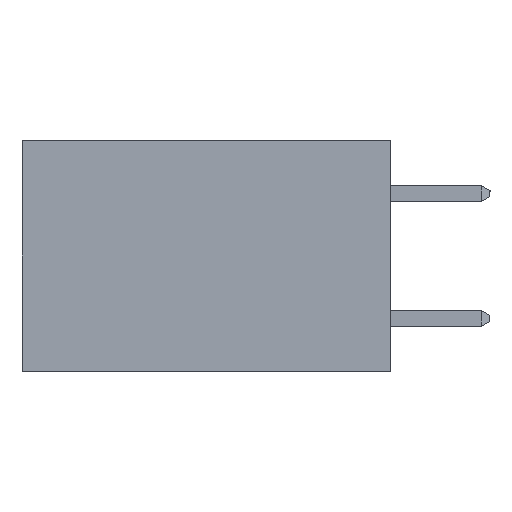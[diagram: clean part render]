
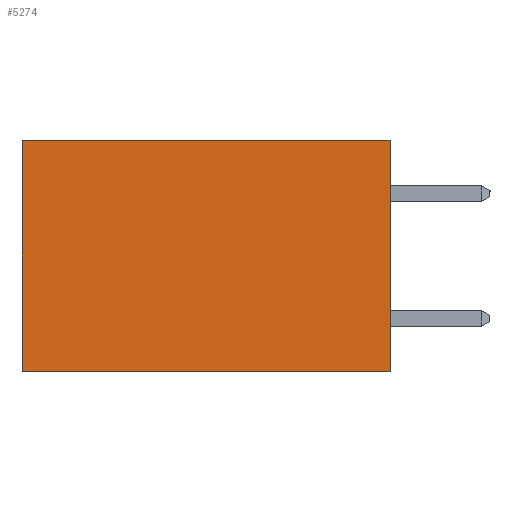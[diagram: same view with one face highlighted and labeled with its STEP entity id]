
A CAD part, left-side view. The second image highlights one B-rep face of the part: STEP entity #5274.
In plain terms, the highlighted planar face has unit normal (-1, 0, 0).
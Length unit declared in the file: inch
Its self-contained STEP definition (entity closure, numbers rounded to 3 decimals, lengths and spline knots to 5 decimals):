
#259 = AXIS2_PLACEMENT_3D ( 'NONE', #12889, #12872, #12855 ) ;
#448 = CARTESIAN_POINT ( 'NONE',  ( 0.277, 0., 0. ) ) ;
#1211 = CARTESIAN_POINT ( 'NONE',  ( 0.277, 0.59, -0.37 ) ) ;
#1327 = EDGE_CURVE ( 'NONE', #5012, #11931, #10814, .T. ) ;
#2160 = EDGE_CURVE ( 'NONE', #11732, #11931, #6467, .T. ) ;
#2224 = ORIENTED_EDGE ( 'NONE', *, *, #1327, .F. ) ;
#2859 = DIRECTION ( 'NONE',  ( 0., 0., -1. ) ) ;
#3295 = EDGE_CURVE ( 'NONE', #13383, #5012, #11925, .T. ) ;
#3427 = CARTESIAN_POINT ( 'NONE',  ( 0.277, 0., -0.37 ) ) ;
#3452 = VECTOR ( 'NONE', #5341, 39.37008 ) ;
#3550 = FACE_OUTER_BOUND ( 'NONE', #4337, .T. ) ;
#4129 = CARTESIAN_POINT ( 'NONE',  ( 0.277, 0.59, 0. ) ) ;
#4337 = EDGE_LOOP ( 'NONE', ( #13172, #2224, #5355, #5174 ) ) ;
#4880 = EDGE_CURVE ( 'NONE', #13383, #11732, #12362, .T. ) ;
#5012 = VERTEX_POINT ( 'NONE', #10967 ) ;
#5174 = ORIENTED_EDGE ( 'NONE', *, *, #4880, .T. ) ;
#5274 = ADVANCED_FACE ( 'NONE', ( #3550 ), #13047, .F. ) ;
#5341 = DIRECTION ( 'NONE',  ( 0., 0., -1. ) ) ;
#5355 = ORIENTED_EDGE ( 'NONE', *, *, #3295, .F. ) ;
#5693 = CARTESIAN_POINT ( 'NONE',  ( 0.277, 0.59, -0.37 ) ) ;
#5754 = VECTOR ( 'NONE', #2859, 39.37008 ) ;
#6467 = LINE ( 'NONE', #5693, #5754 ) ;
#8278 = DIRECTION ( 'NONE',  ( 0., 1., 0. ) ) ;
#8543 = VECTOR ( 'NONE', #8278, 39.37008 ) ;
#10172 = CARTESIAN_POINT ( 'NONE',  ( 0.277, 0., -0.37 ) ) ;
#10472 = VECTOR ( 'NONE', #10936, 39.37008 ) ;
#10814 = LINE ( 'NONE', #10172, #10472 ) ;
#10936 = DIRECTION ( 'NONE',  ( 0., 1., 0. ) ) ;
#10967 = CARTESIAN_POINT ( 'NONE',  ( 0.277, 0., -0.37 ) ) ;
#11732 = VERTEX_POINT ( 'NONE', #4129 ) ;
#11925 = LINE ( 'NONE', #3427, #3452 ) ;
#11931 = VERTEX_POINT ( 'NONE', #1211 ) ;
#12362 = LINE ( 'NONE', #448, #8543 ) ;
#12855 = DIRECTION ( 'NONE',  ( 0., 0., -1. ) ) ;
#12872 = DIRECTION ( 'NONE',  ( 1., 0., 0. ) ) ;
#12889 = CARTESIAN_POINT ( 'NONE',  ( 0.277, 0., -0.37 ) ) ;
#13047 = PLANE ( 'NONE',  #259 ) ;
#13099 = CARTESIAN_POINT ( 'NONE',  ( 0.277, 0., 0. ) ) ;
#13172 = ORIENTED_EDGE ( 'NONE', *, *, #2160, .T. ) ;
#13383 = VERTEX_POINT ( 'NONE', #13099 ) ;
